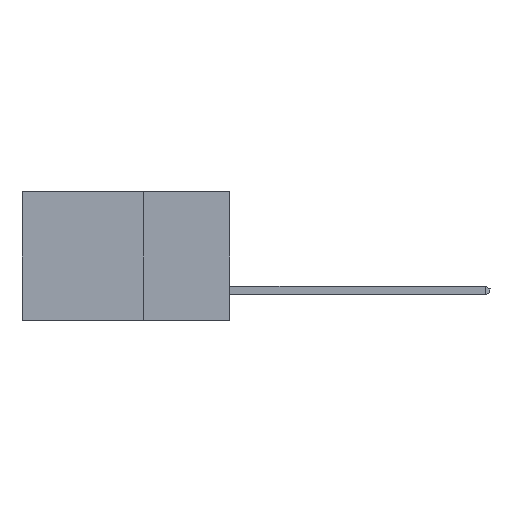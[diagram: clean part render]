
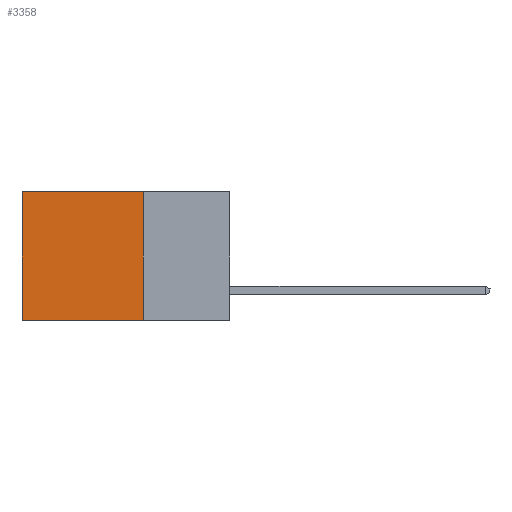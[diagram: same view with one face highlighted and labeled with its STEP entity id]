
A CAD part, left-side view. The second image highlights one B-rep face of the part: STEP entity #3358.
In plain terms, the highlighted planar face has unit normal (-1, 0, 0).
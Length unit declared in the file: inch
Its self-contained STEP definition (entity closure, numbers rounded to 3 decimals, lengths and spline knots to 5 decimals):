
#584 = ORIENTED_EDGE ( 'NONE', *, *, #8092, .T. ) ;
#1037 = DIRECTION ( 'NONE',  ( 0., 0., -1. ) ) ;
#1856 = CARTESIAN_POINT ( 'NONE',  ( 0.2615, 0.25, -0.37 ) ) ;
#1924 = LINE ( 'NONE', #1856, #11351 ) ;
#2320 = VECTOR ( 'NONE', #5807, 39.37008 ) ;
#2350 = EDGE_CURVE ( 'NONE', #11734, #14284, #11272, .T. ) ;
#3066 = CARTESIAN_POINT ( 'NONE',  ( 0.2615, 0.6, -0.37 ) ) ;
#3358 = ADVANCED_FACE ( 'NONE', ( #13954 ), #8400, .F. ) ;
#3572 = CARTESIAN_POINT ( 'NONE',  ( 0.2615, 0.25, 0. ) ) ;
#4470 = DIRECTION ( 'NONE',  ( 0., 0., -1. ) ) ;
#4666 = EDGE_CURVE ( 'NONE', #11734, #7257, #8251, .T. ) ;
#4751 = CARTESIAN_POINT ( 'NONE',  ( 0.2615, 0.25, -0.37 ) ) ;
#4771 = VERTEX_POINT ( 'NONE', #5731 ) ;
#5731 = CARTESIAN_POINT ( 'NONE',  ( 0.2615, 0.6, -0.37 ) ) ;
#5807 = DIRECTION ( 'NONE',  ( 0., 1., 0. ) ) ;
#6410 = VECTOR ( 'NONE', #4470, 39.37008 ) ;
#6547 = LINE ( 'NONE', #3066, #6410 ) ;
#6587 = CARTESIAN_POINT ( 'NONE',  ( 0.2615, 0.25, -0.37 ) ) ;
#6716 = ORIENTED_EDGE ( 'NONE', *, *, #7095, .F. ) ;
#7092 = ORIENTED_EDGE ( 'NONE', *, *, #2350, .F. ) ;
#7095 = EDGE_CURVE ( 'NONE', #14284, #4771, #1924, .T. ) ;
#7207 = CARTESIAN_POINT ( 'NONE',  ( 0.2615, 0.25, 0. ) ) ;
#7257 = VERTEX_POINT ( 'NONE', #7988 ) ;
#7979 = VECTOR ( 'NONE', #1037, 39.37008 ) ;
#7988 = CARTESIAN_POINT ( 'NONE',  ( 0.2615, 0.6, 0. ) ) ;
#8092 = EDGE_CURVE ( 'NONE', #7257, #4771, #6547, .T. ) ;
#8160 = DIRECTION ( 'NONE',  ( 1., 0., 0. ) ) ;
#8229 = DIRECTION ( 'NONE',  ( 0., 0., -1. ) ) ;
#8251 = LINE ( 'NONE', #3572, #2320 ) ;
#8340 = CARTESIAN_POINT ( 'NONE',  ( 0.2615, 0.25, -0.37 ) ) ;
#8400 = PLANE ( 'NONE',  #13224 ) ;
#10654 = ORIENTED_EDGE ( 'NONE', *, *, #4666, .T. ) ;
#10963 = EDGE_LOOP ( 'NONE', ( #584, #6716, #7092, #10654 ) ) ;
#11272 = LINE ( 'NONE', #6587, #7979 ) ;
#11351 = VECTOR ( 'NONE', #14328, 39.37008 ) ;
#11734 = VERTEX_POINT ( 'NONE', #7207 ) ;
#13224 = AXIS2_PLACEMENT_3D ( 'NONE', #4751, #8160, #8229 ) ;
#13954 = FACE_OUTER_BOUND ( 'NONE', #10963, .T. ) ;
#14284 = VERTEX_POINT ( 'NONE', #8340 ) ;
#14328 = DIRECTION ( 'NONE',  ( 0., 1., 0. ) ) ;
